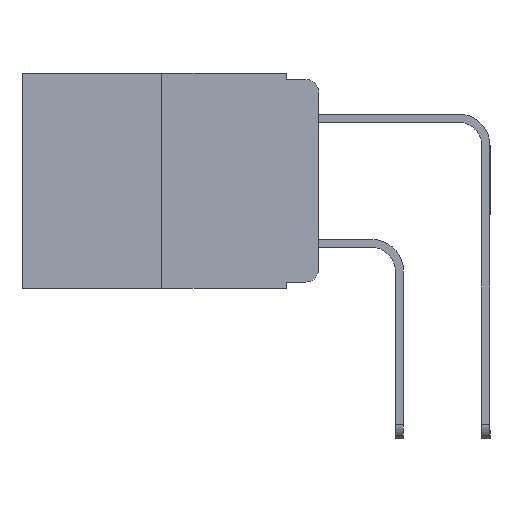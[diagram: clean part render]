
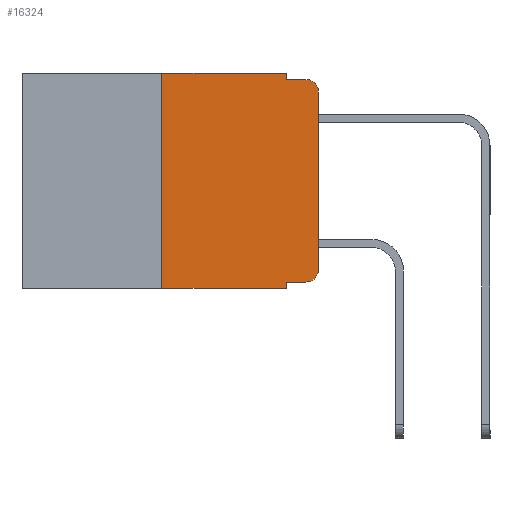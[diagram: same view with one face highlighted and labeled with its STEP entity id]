
A CAD part, left-side view. The second image highlights one B-rep face of the part: STEP entity #16324.
In plain terms, the highlighted planar face has unit normal (-1, 0, 0).
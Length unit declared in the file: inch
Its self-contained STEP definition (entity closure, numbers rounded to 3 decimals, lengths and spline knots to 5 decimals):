
#628 = DIRECTION ( 'NONE',  ( 0., 0., 1. ) ) ;
#1559 = EDGE_CURVE ( 'NONE', #9413, #4939, #8067, .T. ) ;
#1852 = CARTESIAN_POINT ( 'NONE',  ( 0., 0.473, 0. ) ) ;
#2189 = VERTEX_POINT ( 'NONE', #19114 ) ;
#2647 = CARTESIAN_POINT ( 'NONE',  ( 0., 0.473, 0. ) ) ;
#2803 = CARTESIAN_POINT ( 'NONE',  ( 0., 0.051, -0.01 ) ) ;
#2896 = ORIENTED_EDGE ( 'NONE', *, *, #16451, .F. ) ;
#3202 = CARTESIAN_POINT ( 'NONE',  ( 0., 0.25, 0. ) ) ;
#3298 = DIRECTION ( 'NONE',  ( -1., 0., 0. ) ) ;
#3652 = FACE_OUTER_BOUND ( 'NONE', #7840, .T. ) ;
#3738 = LINE ( 'NONE', #8381, #13780 ) ;
#3904 = CARTESIAN_POINT ( 'NONE',  ( 0., 0.02, -0.01 ) ) ;
#4265 = ORIENTED_EDGE ( 'NONE', *, *, #13633, .T. ) ;
#4293 = LINE ( 'NONE', #20841, #20513 ) ;
#4517 = VECTOR ( 'NONE', #18287, 39.37008 ) ;
#4623 = CARTESIAN_POINT ( 'NONE',  ( 0., 0., 0. ) ) ;
#4872 = DIRECTION ( 'NONE',  ( -1., 0., 0. ) ) ;
#4895 = VERTEX_POINT ( 'NONE', #2803 ) ;
#4939 = VERTEX_POINT ( 'NONE', #5213 ) ;
#5148 = VERTEX_POINT ( 'NONE', #24834 ) ;
#5213 = CARTESIAN_POINT ( 'NONE',  ( 0., 0., -0.03 ) ) ;
#5330 = DIRECTION ( 'NONE',  ( 0., -1., 0. ) ) ;
#5470 = VECTOR ( 'NONE', #20400, 39.37008 ) ;
#5974 = CIRCLE ( 'NONE', #8590, 0.02 ) ;
#6134 = DIRECTION ( 'NONE',  ( 0., 0., -1. ) ) ;
#6161 = CARTESIAN_POINT ( 'NONE',  ( 0., 0.25, 0. ) ) ;
#7323 = CARTESIAN_POINT ( 'NONE',  ( 0., 0.473, -0.343 ) ) ;
#7807 = CARTESIAN_POINT ( 'NONE',  ( 0., 0.051, -0.01 ) ) ;
#7840 = EDGE_LOOP ( 'NONE', ( #16585, #22109, #17894, #23395, #13637, #2896, #14276, #20488, #4265, #10671 ) ) ;
#7959 = VECTOR ( 'NONE', #5330, 39.37008 ) ;
#8067 = LINE ( 'NONE', #4623, #13044 ) ;
#8381 = CARTESIAN_POINT ( 'NONE',  ( 0., 0.051, 0. ) ) ;
#8466 = CARTESIAN_POINT ( 'NONE',  ( 0., 0., -0.313 ) ) ;
#8590 = AXIS2_PLACEMENT_3D ( 'NONE', #16094, #3298, #18198 ) ;
#8668 = CIRCLE ( 'NONE', #15941, 0.02 ) ;
#8813 = VERTEX_POINT ( 'NONE', #6161 ) ;
#9413 = VERTEX_POINT ( 'NONE', #8466 ) ;
#9751 = EDGE_CURVE ( 'NONE', #13429, #2189, #25293, .T. ) ;
#10671 = ORIENTED_EDGE ( 'NONE', *, *, #12226, .T. ) ;
#11422 = DIRECTION ( 'NONE',  ( 1., 0., 0. ) ) ;
#12226 = EDGE_CURVE ( 'NONE', #5148, #9413, #8668, .T. ) ;
#12546 = DIRECTION ( 'NONE',  ( 0., 0., -1. ) ) ;
#13044 = VECTOR ( 'NONE', #628, 39.37008 ) ;
#13429 = VERTEX_POINT ( 'NONE', #21639 ) ;
#13633 = EDGE_CURVE ( 'NONE', #13759, #5148, #15837, .T. ) ;
#13637 = ORIENTED_EDGE ( 'NONE', *, *, #13827, .F. ) ;
#13759 = VERTEX_POINT ( 'NONE', #22704 ) ;
#13780 = VECTOR ( 'NONE', #12546, 39.37008 ) ;
#13827 = EDGE_CURVE ( 'NONE', #8813, #15180, #27120, .T. ) ;
#14276 = ORIENTED_EDGE ( 'NONE', *, *, #9751, .T. ) ;
#15028 = EDGE_CURVE ( 'NONE', #13759, #2189, #3738, .T. ) ;
#15180 = VERTEX_POINT ( 'NONE', #17305 ) ;
#15837 = LINE ( 'NONE', #16178, #4517 ) ;
#15941 = AXIS2_PLACEMENT_3D ( 'NONE', #17576, #4872, #19683 ) ;
#16094 = CARTESIAN_POINT ( 'NONE',  ( 0., 0.02, -0.03 ) ) ;
#16178 = CARTESIAN_POINT ( 'NONE',  ( 0., 0.051, -0.333 ) ) ;
#16324 = ADVANCED_FACE ( 'NONE', ( #3652 ), #17658, .F. ) ;
#16451 = EDGE_CURVE ( 'NONE', #13429, #8813, #16655, .T. ) ;
#16585 = ORIENTED_EDGE ( 'NONE', *, *, #1559, .T. ) ;
#16655 = LINE ( 'NONE', #3202, #26971 ) ;
#17305 = CARTESIAN_POINT ( 'NONE',  ( 0., 0.051, 0. ) ) ;
#17576 = CARTESIAN_POINT ( 'NONE',  ( 0., 0.02, -0.313 ) ) ;
#17658 = PLANE ( 'NONE',  #18981 ) ;
#17851 = EDGE_CURVE ( 'NONE', #15180, #4895, #4293, .T. ) ;
#17894 = ORIENTED_EDGE ( 'NONE', *, *, #20615, .F. ) ;
#18198 = DIRECTION ( 'NONE',  ( 0., 0., -1. ) ) ;
#18287 = DIRECTION ( 'NONE',  ( 0., -1., 0. ) ) ;
#18981 = AXIS2_PLACEMENT_3D ( 'NONE', #2647, #11422, #25951 ) ;
#19023 = VERTEX_POINT ( 'NONE', #3904 ) ;
#19114 = CARTESIAN_POINT ( 'NONE',  ( 0., 0.051, -0.343 ) ) ;
#19683 = DIRECTION ( 'NONE',  ( 0., 0., -1. ) ) ;
#20400 = DIRECTION ( 'NONE',  ( 0., -1., 0. ) ) ;
#20488 = ORIENTED_EDGE ( 'NONE', *, *, #15028, .F. ) ;
#20513 = VECTOR ( 'NONE', #6134, 39.37008 ) ;
#20615 = EDGE_CURVE ( 'NONE', #4895, #19023, #22910, .T. ) ;
#20841 = CARTESIAN_POINT ( 'NONE',  ( 0., 0.051, 0. ) ) ;
#21023 = VECTOR ( 'NONE', #23059, 39.37008 ) ;
#21639 = CARTESIAN_POINT ( 'NONE',  ( 0., 0.25, -0.343 ) ) ;
#22109 = ORIENTED_EDGE ( 'NONE', *, *, #26143, .T. ) ;
#22704 = CARTESIAN_POINT ( 'NONE',  ( 0., 0.051, -0.333 ) ) ;
#22910 = LINE ( 'NONE', #7807, #5470 ) ;
#23059 = DIRECTION ( 'NONE',  ( 0., -1., 0. ) ) ;
#23395 = ORIENTED_EDGE ( 'NONE', *, *, #17851, .F. ) ;
#24834 = CARTESIAN_POINT ( 'NONE',  ( 0., 0.02, -0.333 ) ) ;
#25293 = LINE ( 'NONE', #7323, #7959 ) ;
#25951 = DIRECTION ( 'NONE',  ( 0., 0., -1. ) ) ;
#26143 = EDGE_CURVE ( 'NONE', #4939, #19023, #5974, .T. ) ;
#26291 = DIRECTION ( 'NONE',  ( 0., 0., 1. ) ) ;
#26971 = VECTOR ( 'NONE', #26291, 39.37008 ) ;
#27120 = LINE ( 'NONE', #1852, #21023 ) ;
